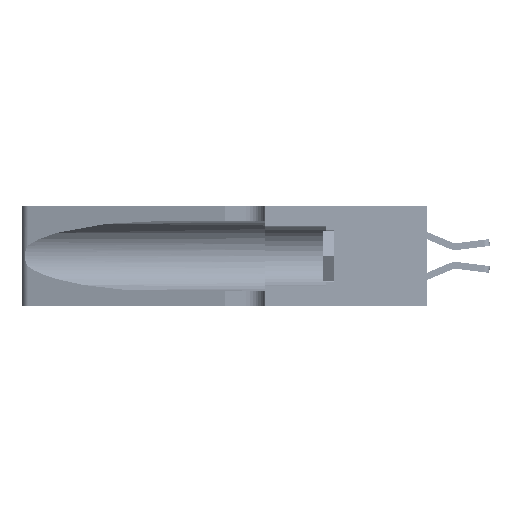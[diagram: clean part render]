
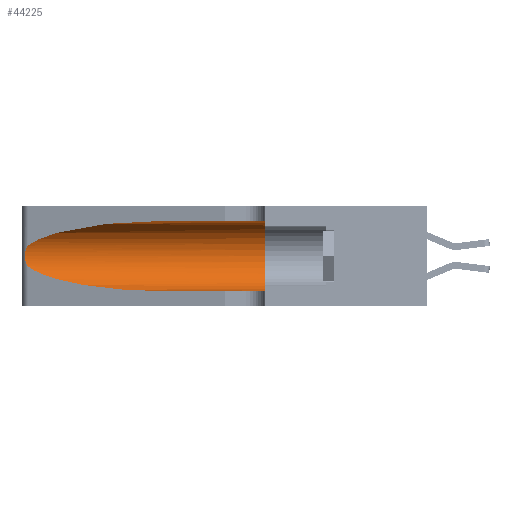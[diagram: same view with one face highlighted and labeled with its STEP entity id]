
A CAD part, left-side view. The second image highlights one B-rep face of the part: STEP entity #44225.
In plain terms, the highlighted cylindrical face has radius 3.308 mm (diameter 6.617 mm), a partial arc.
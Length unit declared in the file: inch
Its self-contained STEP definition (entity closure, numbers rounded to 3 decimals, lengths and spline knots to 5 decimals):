
#555 = CARTESIAN_POINT ( 'NONE',  ( 0.1305, 1.61858, 0.31525 ) ) ;
#688 = CARTESIAN_POINT ( 'NONE',  ( 0.18966, 0.96281, 0.31525 ) ) ;
#1445 = EDGE_CURVE ( 'NONE', #12636, #16976, #13678, .T. ) ;
#1812 = CARTESIAN_POINT ( 'NONE',  ( 0.26017, 1.23833, 0.17102 ) ) ;
#2117 = VECTOR ( 'NONE', #41280, 39.37008 ) ;
#3290 = CARTESIAN_POINT ( 'NONE',  ( 0.2373, 1.15595, 0.08982 ) ) ;
#3296 = LINE ( 'NONE', #30516, #2117 ) ;
#4891 = CARTESIAN_POINT ( 'NONE',  ( 0.1305, 0.35, 0.185 ) ) ;
#5347 = CARTESIAN_POINT ( 'NONE',  ( 0.25487, 1.22718, 0.22369 ) ) ;
#5505 = CARTESIAN_POINT ( 'NONE',  ( 0.25789, 1.23486, 0.15765 ) ) ;
#6819 = CARTESIAN_POINT ( 'NONE',  ( 0.25487, 1.22718, 0.14631 ) ) ;
#8560 = ORIENTED_EDGE ( 'NONE', *, *, #42639, .T. ) ;
#8586 = DIRECTION ( 'NONE',  ( 0., 0., 1. ) ) ;
#9202 = CARTESIAN_POINT ( 'NONE',  ( 0.25555, 1.22993, 0.14849 ) ) ;
#11612 = VERTEX_POINT ( 'NONE', #28412 ) ;
#11731 = AXIS2_PLACEMENT_3D ( 'NONE', #4891, #30118, #8586 ) ;
#12050 = ORIENTED_EDGE ( 'NONE', *, *, #41118, .T. ) ;
#12469 = EDGE_CURVE ( 'NONE', #16976, #28852, #26990, .T. ) ;
#12636 = VERTEX_POINT ( 'NONE', #41632 ) ;
#13678 = LINE ( 'NONE', #555, #41133 ) ;
#14272 = CARTESIAN_POINT ( 'NONE',  ( 0.1305, 0.72297, 0.05475 ) ) ;
#16323 = CARTESIAN_POINT ( 'NONE',  ( 0.25787, 1.23484, 0.2124 ) ) ;
#16976 = VERTEX_POINT ( 'NONE', #28682 ) ;
#17818 = ORIENTED_EDGE ( 'NONE', *, *, #41551, .T. ) ;
#18999 = CARTESIAN_POINT ( 'NONE',  ( 0.2373, 1.15595, 0.28018 ) ) ;
#19993 = CARTESIAN_POINT ( 'NONE',  ( 0.26018, 1.23835, 0.19895 ) ) ;
#22347 = DIRECTION ( 'NONE',  ( 0., -1., 0. ) ) ;
#22953 = VERTEX_POINT ( 'NONE', #6819 ) ;
#23168 = B_SPLINE_CURVE_WITH_KNOTS ( 'NONE', 3,
 ( #5347, #26999, #37749, #16323, #41332, #19993, #44876, #23585, #1812, #27150, #5505, #30719, #9202, #34310 ),
 .UNSPECIFIED., .F., .F.,
 ( 4, 2, 2, 2, 2, 2, 4 ),
 ( 0., 0.00027, 0.00053, 0.00107, 0.0016, 0.00187, 0.00214 ),
 .UNSPECIFIED. ) ;
#23585 = CARTESIAN_POINT ( 'NONE',  ( 0.26075, 1.23896, 0.178 ) ) ;
#23607 = DIRECTION ( 'NONE',  ( 0., 0., -1. ) ) ;
#23799 = ORIENTED_EDGE ( 'NONE', *, *, #1445, .F. ) ;
#25072 = VERTEX_POINT ( 'NONE', #26644 ) ;
#25117 = EDGE_CURVE ( 'NONE', #25072, #28852, #3296, .T. ) ;
#26644 = CARTESIAN_POINT ( 'NONE',  ( 0.1305, 0.72297, 0.05475 ) ) ;
#26990 = CIRCLE ( 'NONE', #11731, 0.13025 ) ;
#26999 = CARTESIAN_POINT ( 'NONE',  ( 0.25555, 1.22994, 0.2215 ) ) ;
#27150 = CARTESIAN_POINT ( 'NONE',  ( 0.25856, 1.23593, 0.16098 ) ) ;
#28001 =( BOUNDED_CURVE ( )  B_SPLINE_CURVE ( 3, ( #33180, #688, #18999, #43908 ),
 .UNSPECIFIED., .F., .F. ) 
 B_SPLINE_CURVE_WITH_KNOTS ( ( 4, 4 ),
 ( 1.5708, 2.84003 ),
 .UNSPECIFIED. ) 
 CURVE ( )  GEOMETRIC_REPRESENTATION_ITEM ( )  RATIONAL_B_SPLINE_CURVE ( ( 1., 0.87, 0.87, 1. ) ) 
 REPRESENTATION_ITEM ( '' )  );
#28412 = CARTESIAN_POINT ( 'NONE',  ( 0.25487, 1.22718, 0.22369 ) ) ;
#28441 = FACE_OUTER_BOUND ( 'NONE', #30176, .T. ) ;
#28682 = CARTESIAN_POINT ( 'NONE',  ( 0.1305, 0.35, 0.31525 ) ) ;
#28761 = CARTESIAN_POINT ( 'NONE',  ( 0.1305, 0.35, 0.05475 ) ) ;
#28852 = VERTEX_POINT ( 'NONE', #28761 ) ;
#28857 =( BOUNDED_CURVE ( )  B_SPLINE_CURVE ( 3, ( #32140, #3290, #35749, #14272 ),
 .UNSPECIFIED., .F., .F. ) 
 B_SPLINE_CURVE_WITH_KNOTS ( ( 4, 4 ),
 ( 3.44316, 4.71239 ),
 .UNSPECIFIED. ) 
 CURVE ( )  GEOMETRIC_REPRESENTATION_ITEM ( )  RATIONAL_B_SPLINE_CURVE ( ( 1., 0.87, 0.87, 1. ) ) 
 REPRESENTATION_ITEM ( '' )  );
#30118 = DIRECTION ( 'NONE',  ( 0., 1., 0. ) ) ;
#30176 = EDGE_LOOP ( 'NONE', ( #17818, #12050, #8560, #41681, #45903, #23799 ) ) ;
#30516 = CARTESIAN_POINT ( 'NONE',  ( 0.1305, 1.61858, 0.05475 ) ) ;
#30719 = CARTESIAN_POINT ( 'NONE',  ( 0.25639, 1.23186, 0.15144 ) ) ;
#32140 = CARTESIAN_POINT ( 'NONE',  ( 0.25487, 1.22718, 0.14631 ) ) ;
#33180 = CARTESIAN_POINT ( 'NONE',  ( 0.1305, 0.72297, 0.31525 ) ) ;
#34310 = CARTESIAN_POINT ( 'NONE',  ( 0.25487, 1.22718, 0.14631 ) ) ;
#34554 = CYLINDRICAL_SURFACE ( 'NONE', #46479, 0.13025 ) ;
#35749 = CARTESIAN_POINT ( 'NONE',  ( 0.18966, 0.96281, 0.05475 ) ) ;
#37749 = CARTESIAN_POINT ( 'NONE',  ( 0.25639, 1.23184, 0.21858 ) ) ;
#41118 = EDGE_CURVE ( 'NONE', #11612, #22953, #23168, .T. ) ;
#41133 = VECTOR ( 'NONE', #22347, 39.37008 ) ;
#41280 = DIRECTION ( 'NONE',  ( 0., -1., 0. ) ) ;
#41332 = CARTESIAN_POINT ( 'NONE',  ( 0.25854, 1.2359, 0.20912 ) ) ;
#41346 = CARTESIAN_POINT ( 'NONE',  ( 0.1305, 1.61858, 0.185 ) ) ;
#41551 = EDGE_CURVE ( 'NONE', #12636, #11612, #28001, .T. ) ;
#41632 = CARTESIAN_POINT ( 'NONE',  ( 0.1305, 0.72297, 0.31525 ) ) ;
#41681 = ORIENTED_EDGE ( 'NONE', *, *, #25117, .T. ) ;
#42639 = EDGE_CURVE ( 'NONE', #22953, #25072, #28857, .T. ) ;
#43908 = CARTESIAN_POINT ( 'NONE',  ( 0.25487, 1.22718, 0.22369 ) ) ;
#44225 = ADVANCED_FACE ( 'NONE', ( #28441 ), #34554, .F. ) ;
#44876 = CARTESIAN_POINT ( 'NONE',  ( 0.26075, 1.23896, 0.19203 ) ) ;
#44892 = DIRECTION ( 'NONE',  ( 0., -1., 0. ) ) ;
#45903 = ORIENTED_EDGE ( 'NONE', *, *, #12469, .F. ) ;
#46479 = AXIS2_PLACEMENT_3D ( 'NONE', #41346, #44892, #23607 ) ;
